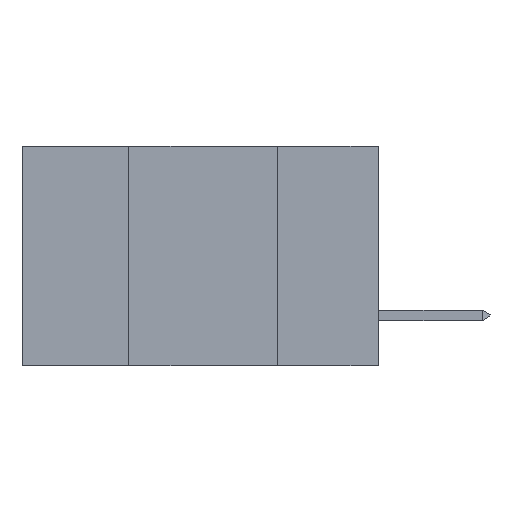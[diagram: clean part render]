
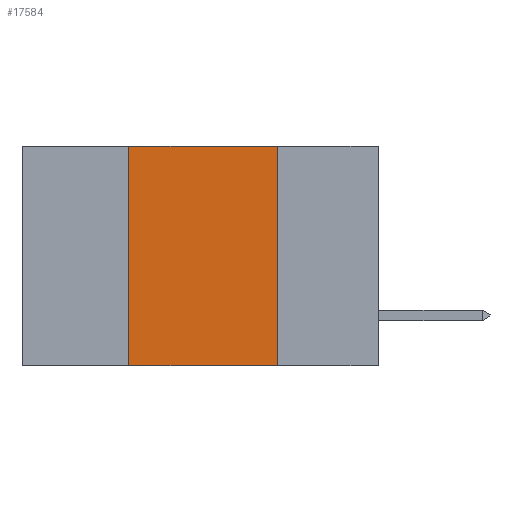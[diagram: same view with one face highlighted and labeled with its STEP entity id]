
A CAD part, left-side view. The second image highlights one B-rep face of the part: STEP entity #17584.
In plain terms, the highlighted planar face has unit normal (-1, 0, 0).
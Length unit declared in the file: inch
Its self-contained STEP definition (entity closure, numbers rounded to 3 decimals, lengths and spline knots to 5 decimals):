
#433 = EDGE_CURVE ( 'NONE', #1999, #9977, #17378, .T. ) ;
#624 = DIRECTION ( 'NONE',  ( 0., -1., 0. ) ) ;
#981 = DIRECTION ( 'NONE',  ( 0., 0., -1. ) ) ;
#1999 = VERTEX_POINT ( 'NONE', #19182 ) ;
#2360 = CARTESIAN_POINT ( 'NONE',  ( 0., 0.6, -0.37 ) ) ;
#2788 = CARTESIAN_POINT ( 'NONE',  ( 0., 0.6, 0. ) ) ;
#3038 = LINE ( 'NONE', #23457, #5652 ) ;
#5652 = VECTOR ( 'NONE', #8915, 39.37008 ) ;
#5707 = DIRECTION ( 'NONE',  ( 0., 0., -1. ) ) ;
#5799 = VECTOR ( 'NONE', #5707, 39.37008 ) ;
#6465 = EDGE_CURVE ( 'NONE', #1999, #11296, #3038, .T. ) ;
#6687 = AXIS2_PLACEMENT_3D ( 'NONE', #2788, #21353, #981 ) ;
#6707 = LINE ( 'NONE', #12973, #20867 ) ;
#8915 = DIRECTION ( 'NONE',  ( 0., 0., 1. ) ) ;
#9044 = VECTOR ( 'NONE', #624, 39.37008 ) ;
#9658 = ORIENTED_EDGE ( 'NONE', *, *, #16954, .F. ) ;
#9977 = VERTEX_POINT ( 'NONE', #15282 ) ;
#11012 = ORIENTED_EDGE ( 'NONE', *, *, #433, .T. ) ;
#11296 = VERTEX_POINT ( 'NONE', #19362 ) ;
#12944 = CARTESIAN_POINT ( 'NONE',  ( 0., 0.17, 0. ) ) ;
#12973 = CARTESIAN_POINT ( 'NONE',  ( 0., 0.6, 0. ) ) ;
#14479 = FACE_OUTER_BOUND ( 'NONE', #21403, .T. ) ;
#15282 = CARTESIAN_POINT ( 'NONE',  ( 0., 0.17, -0.37 ) ) ;
#15376 = LINE ( 'NONE', #18601, #5799 ) ;
#15586 = PLANE ( 'NONE',  #6687 ) ;
#16285 = EDGE_CURVE ( 'NONE', #11296, #16990, #6707, .T. ) ;
#16767 = DIRECTION ( 'NONE',  ( 0., -1., 0. ) ) ;
#16954 = EDGE_CURVE ( 'NONE', #16990, #9977, #15376, .T. ) ;
#16990 = VERTEX_POINT ( 'NONE', #12944 ) ;
#17378 = LINE ( 'NONE', #2360, #9044 ) ;
#17584 = ADVANCED_FACE ( 'NONE', ( #14479 ), #15586, .F. ) ;
#18601 = CARTESIAN_POINT ( 'NONE',  ( 0., 0.17, 0. ) ) ;
#19182 = CARTESIAN_POINT ( 'NONE',  ( 0., 0.42, -0.37 ) ) ;
#19362 = CARTESIAN_POINT ( 'NONE',  ( 0., 0.42, 0. ) ) ;
#20785 = ORIENTED_EDGE ( 'NONE', *, *, #16285, .F. ) ;
#20867 = VECTOR ( 'NONE', #16767, 39.37008 ) ;
#21353 = DIRECTION ( 'NONE',  ( 1., 0., 0. ) ) ;
#21403 = EDGE_LOOP ( 'NONE', ( #9658, #20785, #23091, #11012 ) ) ;
#23091 = ORIENTED_EDGE ( 'NONE', *, *, #6465, .F. ) ;
#23457 = CARTESIAN_POINT ( 'NONE',  ( 0., 0.42, 0. ) ) ;
